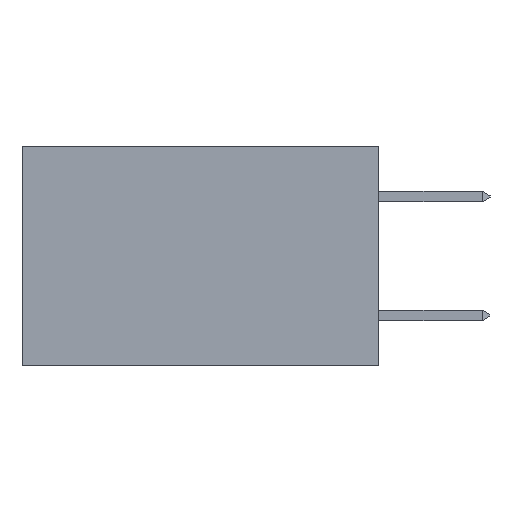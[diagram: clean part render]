
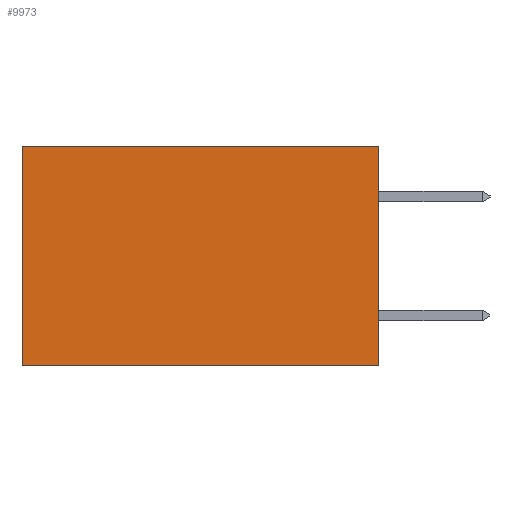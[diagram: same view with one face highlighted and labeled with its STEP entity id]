
A CAD part, left-side view. The second image highlights one B-rep face of the part: STEP entity #9973.
In plain terms, the highlighted planar face has unit normal (-1, 0, 0).
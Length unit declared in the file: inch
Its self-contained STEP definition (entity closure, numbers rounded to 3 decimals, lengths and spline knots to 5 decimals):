
#261 = VECTOR ( 'NONE', #4431, 39.37008 ) ;
#423 = EDGE_LOOP ( 'NONE', ( #4452, #13177, #8738, #3351 ) ) ;
#1608 = EDGE_CURVE ( 'NONE', #4592, #13422, #5992, .T. ) ;
#1879 = PLANE ( 'NONE',  #11776 ) ;
#3351 = ORIENTED_EDGE ( 'NONE', *, *, #1608, .T. ) ;
#3597 = CARTESIAN_POINT ( 'NONE',  ( 0.298, 0., -0.37 ) ) ;
#4383 = CARTESIAN_POINT ( 'NONE',  ( 0.298, 0., -0.37 ) ) ;
#4431 = DIRECTION ( 'NONE',  ( 0., 0., -1. ) ) ;
#4436 = VERTEX_POINT ( 'NONE', #8877 ) ;
#4452 = ORIENTED_EDGE ( 'NONE', *, *, #5939, .T. ) ;
#4509 = CARTESIAN_POINT ( 'NONE',  ( 0.298, 0., 0. ) ) ;
#4592 = VERTEX_POINT ( 'NONE', #6889 ) ;
#4685 = FACE_OUTER_BOUND ( 'NONE', #423, .T. ) ;
#4912 = DIRECTION ( 'NONE',  ( 0., 1., 0. ) ) ;
#5735 = LINE ( 'NONE', #8916, #11019 ) ;
#5939 = EDGE_CURVE ( 'NONE', #13422, #4436, #5735, .T. ) ;
#5992 = LINE ( 'NONE', #10775, #9493 ) ;
#6174 = VECTOR ( 'NONE', #11489, 39.37008 ) ;
#6569 = VERTEX_POINT ( 'NONE', #4383 ) ;
#6769 = DIRECTION ( 'NONE',  ( 1., 0., 0. ) ) ;
#6889 = CARTESIAN_POINT ( 'NONE',  ( 0.298, 0., 0. ) ) ;
#8249 = DIRECTION ( 'NONE',  ( 0., 0., -1. ) ) ;
#8260 = CARTESIAN_POINT ( 'NONE',  ( 0.298, 0.6, 0. ) ) ;
#8738 = ORIENTED_EDGE ( 'NONE', *, *, #11545, .F. ) ;
#8877 = CARTESIAN_POINT ( 'NONE',  ( 0.298, 0.6, -0.37 ) ) ;
#8916 = CARTESIAN_POINT ( 'NONE',  ( 0.298, 0.6, 0. ) ) ;
#8987 = LINE ( 'NONE', #3597, #6174 ) ;
#9240 = DIRECTION ( 'NONE',  ( 0., 0., -1. ) ) ;
#9377 = EDGE_CURVE ( 'NONE', #6569, #4436, #8987, .T. ) ;
#9493 = VECTOR ( 'NONE', #4912, 39.37008 ) ;
#9973 = ADVANCED_FACE ( 'NONE', ( #4685 ), #1879, .F. ) ;
#10775 = CARTESIAN_POINT ( 'NONE',  ( 0.298, 0., 0. ) ) ;
#11019 = VECTOR ( 'NONE', #9240, 39.37008 ) ;
#11335 = LINE ( 'NONE', #4509, #261 ) ;
#11489 = DIRECTION ( 'NONE',  ( 0., 1., 0. ) ) ;
#11545 = EDGE_CURVE ( 'NONE', #4592, #6569, #11335, .T. ) ;
#11776 = AXIS2_PLACEMENT_3D ( 'NONE', #11777, #6769, #8249 ) ;
#11777 = CARTESIAN_POINT ( 'NONE',  ( 0.298, 0., 0. ) ) ;
#13177 = ORIENTED_EDGE ( 'NONE', *, *, #9377, .F. ) ;
#13422 = VERTEX_POINT ( 'NONE', #8260 ) ;
